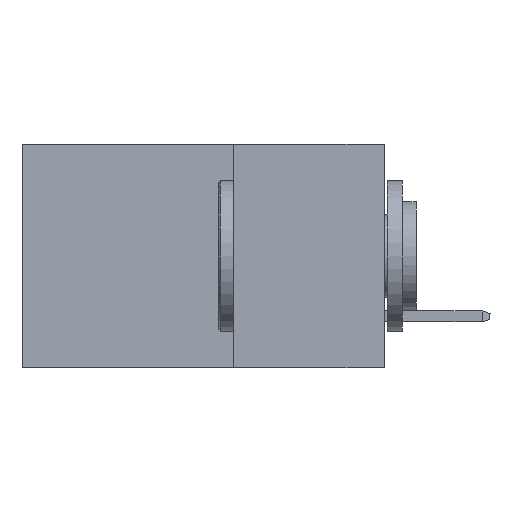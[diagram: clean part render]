
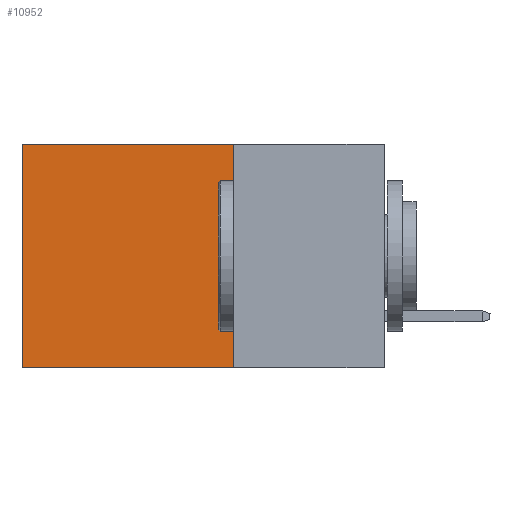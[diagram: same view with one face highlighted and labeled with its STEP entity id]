
A CAD part, left-side view. The second image highlights one B-rep face of the part: STEP entity #10952.
In plain terms, the highlighted planar face has unit normal (-1, 0, 0).
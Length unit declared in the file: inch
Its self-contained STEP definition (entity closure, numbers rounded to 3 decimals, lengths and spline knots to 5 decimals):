
#203 = VERTEX_POINT ( 'NONE', #19080 ) ;
#649 = EDGE_CURVE ( 'NONE', #12661, #203, #13446, .T. ) ;
#1325 = VERTEX_POINT ( 'NONE', #21618 ) ;
#1532 = ORIENTED_EDGE ( 'NONE', *, *, #649, .F. ) ;
#2339 = VECTOR ( 'NONE', #10247, 39.37008 ) ;
#4322 = DIRECTION ( 'NONE',  ( 0., 0., -1. ) ) ;
#4970 = EDGE_CURVE ( 'NONE', #13270, #1325, #14061, .T. ) ;
#6119 = LINE ( 'NONE', #13342, #17168 ) ;
#6356 = AXIS2_PLACEMENT_3D ( 'NONE', #9132, #9243, #13027 ) ;
#7116 = FACE_OUTER_BOUND ( 'NONE', #23127, .T. ) ;
#7118 = ORIENTED_EDGE ( 'NONE', *, *, #18916, .F. ) ;
#9132 = CARTESIAN_POINT ( 'NONE',  ( 0.2615, 0.25, -0.37 ) ) ;
#9161 = ORIENTED_EDGE ( 'NONE', *, *, #12179, .T. ) ;
#9243 = DIRECTION ( 'NONE',  ( 1., 0., 0. ) ) ;
#10247 = DIRECTION ( 'NONE',  ( 0., 1., 0. ) ) ;
#10330 = LINE ( 'NONE', #15794, #12047 ) ;
#10952 = ADVANCED_FACE ( 'NONE', ( #7116 ), #14586, .F. ) ;
#12047 = VECTOR ( 'NONE', #23072, 39.37008 ) ;
#12179 = EDGE_CURVE ( 'NONE', #1325, #203, #10330, .T. ) ;
#12661 = VERTEX_POINT ( 'NONE', #15763 ) ;
#13027 = DIRECTION ( 'NONE',  ( 0., 0., -1. ) ) ;
#13270 = VERTEX_POINT ( 'NONE', #16625 ) ;
#13342 = CARTESIAN_POINT ( 'NONE',  ( 0.2615, 0.25, -0.37 ) ) ;
#13446 = LINE ( 'NONE', #13677, #2339 ) ;
#13677 = CARTESIAN_POINT ( 'NONE',  ( 0.2615, 0.25, -0.37 ) ) ;
#14061 = LINE ( 'NONE', #21810, #18350 ) ;
#14586 = PLANE ( 'NONE',  #6356 ) ;
#15763 = CARTESIAN_POINT ( 'NONE',  ( 0.2615, 0.25, -0.37 ) ) ;
#15794 = CARTESIAN_POINT ( 'NONE',  ( 0.2615, 0.6, -0.37 ) ) ;
#16625 = CARTESIAN_POINT ( 'NONE',  ( 0.2615, 0.25, 0. ) ) ;
#17168 = VECTOR ( 'NONE', #4322, 39.37008 ) ;
#17645 = DIRECTION ( 'NONE',  ( 0., 1., 0. ) ) ;
#17650 = ORIENTED_EDGE ( 'NONE', *, *, #4970, .T. ) ;
#18350 = VECTOR ( 'NONE', #17645, 39.37008 ) ;
#18916 = EDGE_CURVE ( 'NONE', #13270, #12661, #6119, .T. ) ;
#19080 = CARTESIAN_POINT ( 'NONE',  ( 0.2615, 0.6, -0.37 ) ) ;
#21618 = CARTESIAN_POINT ( 'NONE',  ( 0.2615, 0.6, 0. ) ) ;
#21810 = CARTESIAN_POINT ( 'NONE',  ( 0.2615, 0.25, 0. ) ) ;
#23072 = DIRECTION ( 'NONE',  ( 0., 0., -1. ) ) ;
#23127 = EDGE_LOOP ( 'NONE', ( #9161, #1532, #7118, #17650 ) ) ;
